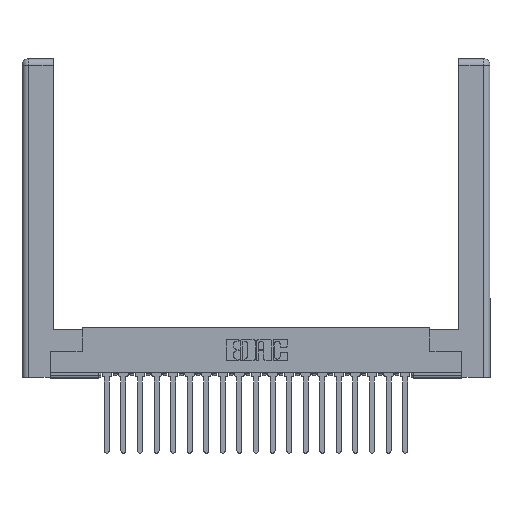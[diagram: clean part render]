
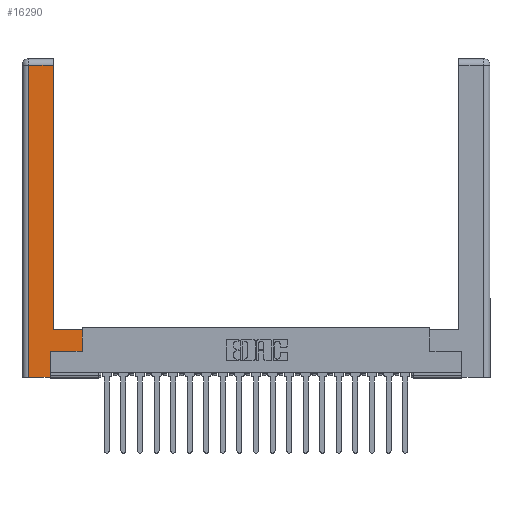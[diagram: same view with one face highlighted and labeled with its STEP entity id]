
A CAD part, top view. The second image highlights one B-rep face of the part: STEP entity #16290.
In plain terms, the highlighted planar face has unit normal (0, 0, 1).
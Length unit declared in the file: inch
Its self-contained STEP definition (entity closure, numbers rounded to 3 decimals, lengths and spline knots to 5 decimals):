
#277 = CARTESIAN_POINT ( 'NONE',  ( 0.0615, 0., 0. ) ) ;
#569 = DIRECTION ( 'NONE',  ( 0., 1., 0. ) ) ;
#1282 = DIRECTION ( 'NONE',  ( -1., 0., 0. ) ) ;
#1482 = VERTEX_POINT ( 'NONE', #17177 ) ;
#1675 = EDGE_LOOP ( 'NONE', ( #9512, #17367, #17982, #9525, #2644, #20261, #20469, #13969 ) ) ;
#1713 = VECTOR ( 'NONE', #16470, 39.37008 ) ;
#1726 = VERTEX_POINT ( 'NONE', #6792 ) ;
#2210 = LINE ( 'NONE', #8927, #2451 ) ;
#2451 = VECTOR ( 'NONE', #569, 39.37008 ) ;
#2644 = ORIENTED_EDGE ( 'NONE', *, *, #20510, .T. ) ;
#2796 = LINE ( 'NONE', #11061, #8879 ) ;
#2819 = VECTOR ( 'NONE', #18267, 39.37008 ) ;
#3100 = CARTESIAN_POINT ( 'NONE',  ( 0.0615, 0., 0. ) ) ;
#3524 = LINE ( 'NONE', #10234, #4306 ) ;
#3661 = EDGE_CURVE ( 'NONE', #6375, #8738, #2796, .T. ) ;
#3670 = CARTESIAN_POINT ( 'NONE',  ( 0.295, 2.94, 0. ) ) ;
#3676 = VERTEX_POINT ( 'NONE', #17868 ) ;
#4306 = VECTOR ( 'NONE', #16940, 39.37008 ) ;
#4677 = LINE ( 'NONE', #12939, #5659 ) ;
#4905 = CARTESIAN_POINT ( 'NONE',  ( 0., 0., 0. ) ) ;
#5659 = VECTOR ( 'NONE', #11601, 39.37008 ) ;
#6290 = LINE ( 'NONE', #3100, #2819 ) ;
#6357 = LINE ( 'NONE', #14722, #1713 ) ;
#6375 = VERTEX_POINT ( 'NONE', #3670 ) ;
#6443 = PLANE ( 'NONE',  #16953 ) ;
#6792 = CARTESIAN_POINT ( 'NONE',  ( 0.565, 0.245, 0. ) ) ;
#7628 = CARTESIAN_POINT ( 'NONE',  ( 0.265, 0., 0. ) ) ;
#8203 = DIRECTION ( 'NONE',  ( 0., 0., -1. ) ) ;
#8315 = FACE_OUTER_BOUND ( 'NONE', #1675, .T. ) ;
#8325 = EDGE_CURVE ( 'NONE', #1482, #6375, #6357, .T. ) ;
#8738 = VERTEX_POINT ( 'NONE', #11806 ) ;
#8879 = VECTOR ( 'NONE', #19298, 39.37008 ) ;
#8927 = CARTESIAN_POINT ( 'NONE',  ( 0.265, 0.245, 0. ) ) ;
#9152 = VECTOR ( 'NONE', #15468, 39.37008 ) ;
#9512 = ORIENTED_EDGE ( 'NONE', *, *, #8325, .T. ) ;
#9525 = ORIENTED_EDGE ( 'NONE', *, *, #19084, .T. ) ;
#10139 = VERTEX_POINT ( 'NONE', #277 ) ;
#10234 = CARTESIAN_POINT ( 'NONE',  ( 0.265, 0., 0. ) ) ;
#10261 = CARTESIAN_POINT ( 'NONE',  ( 0.565, 0.245, 0. ) ) ;
#10407 = LINE ( 'NONE', #11549, #9152 ) ;
#11061 = CARTESIAN_POINT ( 'NONE',  ( 0.0615, 2.94, 0. ) ) ;
#11549 = CARTESIAN_POINT ( 'NONE',  ( 0.295, 0.45, 0. ) ) ;
#11601 = DIRECTION ( 'NONE',  ( 0., 1., 0. ) ) ;
#11806 = CARTESIAN_POINT ( 'NONE',  ( 0.0615, 2.94, 0. ) ) ;
#12939 = CARTESIAN_POINT ( 'NONE',  ( 0.565, 0.45, 0. ) ) ;
#13969 = ORIENTED_EDGE ( 'NONE', *, *, #19441, .T. ) ;
#14402 = EDGE_CURVE ( 'NONE', #8738, #10139, #6290, .T. ) ;
#14722 = CARTESIAN_POINT ( 'NONE',  ( 0.295, 3., 0. ) ) ;
#15425 = EDGE_CURVE ( 'NONE', #19301, #1726, #20285, .T. ) ;
#15468 = DIRECTION ( 'NONE',  ( -1., 0., 0. ) ) ;
#15475 = VERTEX_POINT ( 'NONE', #7628 ) ;
#16290 = ADVANCED_FACE ( 'NONE', ( #8315 ), #6443, .F. ) ;
#16470 = DIRECTION ( 'NONE',  ( 0., 1., 0. ) ) ;
#16895 = VECTOR ( 'NONE', #18728, 39.37008 ) ;
#16940 = DIRECTION ( 'NONE',  ( 1., 0., 0. ) ) ;
#16953 = AXIS2_PLACEMENT_3D ( 'NONE', #4905, #8203, #1282 ) ;
#17177 = CARTESIAN_POINT ( 'NONE',  ( 0.295, 0.45, 0. ) ) ;
#17367 = ORIENTED_EDGE ( 'NONE', *, *, #3661, .T. ) ;
#17868 = CARTESIAN_POINT ( 'NONE',  ( 0.565, 0.45, 0. ) ) ;
#17982 = ORIENTED_EDGE ( 'NONE', *, *, #14402, .T. ) ;
#18267 = DIRECTION ( 'NONE',  ( 0., -1., 0. ) ) ;
#18728 = DIRECTION ( 'NONE',  ( 1., 0., 0. ) ) ;
#19084 = EDGE_CURVE ( 'NONE', #10139, #15475, #3524, .T. ) ;
#19298 = DIRECTION ( 'NONE',  ( -1., 0., 0. ) ) ;
#19301 = VERTEX_POINT ( 'NONE', #21225 ) ;
#19441 = EDGE_CURVE ( 'NONE', #3676, #1482, #10407, .T. ) ;
#19734 = EDGE_CURVE ( 'NONE', #1726, #3676, #4677, .T. ) ;
#20261 = ORIENTED_EDGE ( 'NONE', *, *, #15425, .T. ) ;
#20285 = LINE ( 'NONE', #10261, #16895 ) ;
#20469 = ORIENTED_EDGE ( 'NONE', *, *, #19734, .T. ) ;
#20510 = EDGE_CURVE ( 'NONE', #15475, #19301, #2210, .T. ) ;
#21225 = CARTESIAN_POINT ( 'NONE',  ( 0.265, 0.245, 0. ) ) ;
